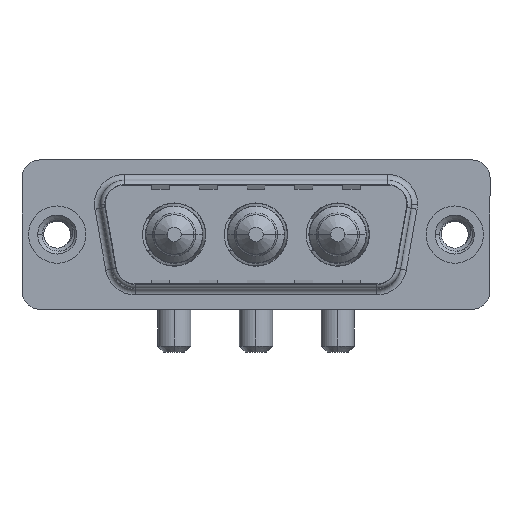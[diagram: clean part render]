
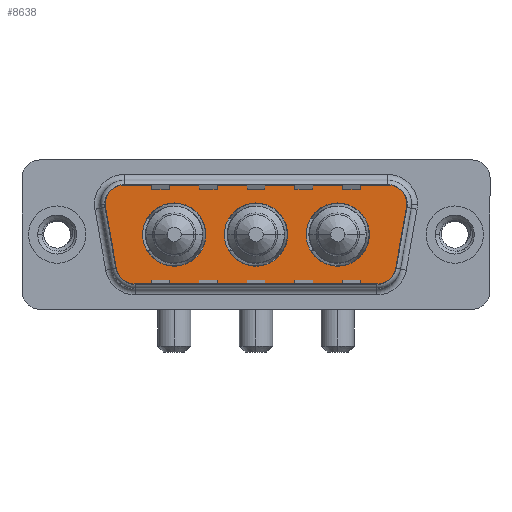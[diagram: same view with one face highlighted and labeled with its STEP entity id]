
A CAD part, top view. The second image highlights one B-rep face of the part: STEP entity #8638.
In plain terms, the highlighted planar face has unit normal (0, 0, 1).
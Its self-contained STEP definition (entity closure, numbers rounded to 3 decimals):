
#4 = CARTESIAN_POINT ( 'NONE',  ( 5.411, 2.9, 0. ) ) ;
#102 = EDGE_CURVE ( 'NONE', #4519, #10215, #9988, .T. ) ;
#134 = CARTESIAN_POINT ( 'NONE',  ( 5.411, 4.9, 0. ) ) ;
#168 = DIRECTION ( 'NONE',  ( 1., 0., 0. ) ) ;
#295 = CIRCLE ( 'NONE', #10770, 2. ) ;
#308 = DIRECTION ( 'NONE',  ( 1., 0., 0. ) ) ;
#319 = LINE ( 'NONE', #379, #3929 ) ;
#379 = CARTESIAN_POINT ( 'NONE',  ( 3.441, 2.553, 0. ) ) ;
#407 = EDGE_LOOP ( 'NONE', ( #12001, #1550 ) ) ;
#461 = EDGE_CURVE ( 'NONE', #5105, #5232, #768, .T. ) ;
#564 = VERTEX_POINT ( 'NONE', #7738 ) ;
#615 = DIRECTION ( 'NONE',  ( 0., 0., 1. ) ) ;
#768 = CIRCLE ( 'NONE', #2025, 2.65 ) ;
#1009 = ORIENTED_EDGE ( 'NONE', *, *, #1290, .T. ) ;
#1150 = CARTESIAN_POINT ( 'NONE',  ( 9.8, 0., 0. ) ) ;
#1290 = EDGE_CURVE ( 'NONE', #6706, #10759, #6469, .T. ) ;
#1369 = EDGE_LOOP ( 'NONE', ( #8035, #1009, #5273, #9855, #12425, #7661, #12326, #8257, #8322 ) ) ;
#1381 = DIRECTION ( 'NONE',  ( 1., 0., 0. ) ) ;
#1436 = DIRECTION ( 'NONE',  ( 1., 0., 0. ) ) ;
#1550 = ORIENTED_EDGE ( 'NONE', *, *, #9164, .F. ) ;
#1664 = CARTESIAN_POINT ( 'NONE',  ( 27.889, 2.9, 0. ) ) ;
#1695 = DIRECTION ( 'NONE',  ( 1., 0., 0. ) ) ;
#1809 = EDGE_CURVE ( 'NONE', #5110, #6706, #10409, .T. ) ;
#2025 = AXIS2_PLACEMENT_3D ( 'NONE', #12736, #9695, #1695 ) ;
#2200 = FACE_BOUND ( 'NONE', #7278, .T. ) ;
#2333 = EDGE_CURVE ( 'NONE', #10215, #7898, #319, .T. ) ;
#2494 = ORIENTED_EDGE ( 'NONE', *, *, #5559, .F. ) ;
#2675 = DIRECTION ( 'NONE',  ( -1., 0., 0. ) ) ;
#2736 = VERTEX_POINT ( 'NONE', #4322 ) ;
#3080 = CARTESIAN_POINT ( 'NONE',  ( 5.411, 4.9, 0. ) ) ;
#3264 = CARTESIAN_POINT ( 'NONE',  ( 26.15, 0., 0. ) ) ;
#3303 = AXIS2_PLACEMENT_3D ( 'NONE', #10310, #6513, #1381 ) ;
#3360 = EDGE_CURVE ( 'NONE', #8669, #5110, #3575, .T. ) ;
#3575 = LINE ( 'NONE', #11386, #5427 ) ;
#3820 = AXIS2_PLACEMENT_3D ( 'NONE', #5224, #9296, #308 ) ;
#3929 = VECTOR ( 'NONE', #7408, 1000. ) ;
#4125 = DIRECTION ( 'NONE',  ( 0., 0., 1. ) ) ;
#4252 = AXIS2_PLACEMENT_3D ( 'NONE', #1150, #4295, #168 ) ;
#4295 = DIRECTION ( 'NONE',  ( 0., 0., 1. ) ) ;
#4322 = CARTESIAN_POINT ( 'NONE',  ( 19.3, 0., 0. ) ) ;
#4519 = VERTEX_POINT ( 'NONE', #3080 ) ;
#4609 = CARTESIAN_POINT ( 'NONE',  ( 6.434, -2.9, 0. ) ) ;
#4753 = AXIS2_PLACEMENT_3D ( 'NONE', #5583, #12183, #9575 ) ;
#4786 = CIRCLE ( 'NONE', #9814, 2. ) ;
#5051 = DIRECTION ( 'NONE',  ( -1., 0., 0. ) ) ;
#5105 = VERTEX_POINT ( 'NONE', #9562 ) ;
#5110 = VERTEX_POINT ( 'NONE', #7670 ) ;
#5224 = CARTESIAN_POINT ( 'NONE',  ( 26.866, -2.9, 0. ) ) ;
#5232 = VERTEX_POINT ( 'NONE', #8582 ) ;
#5273 = ORIENTED_EDGE ( 'NONE', *, *, #9786, .T. ) ;
#5292 = FACE_OUTER_BOUND ( 'NONE', #1369, .T. ) ;
#5427 = VECTOR ( 'NONE', #1436, 1000. ) ;
#5540 = DIRECTION ( 'NONE',  ( 1., 0., 0. ) ) ;
#5559 = EDGE_CURVE ( 'NONE', #5232, #5105, #12180, .T. ) ;
#5583 = CARTESIAN_POINT ( 'NONE',  ( 26.866, -2.9, 0. ) ) ;
#5640 = CIRCLE ( 'NONE', #3303, 2.65 ) ;
#5834 = VECTOR ( 'NONE', #11415, 1000. ) ;
#5925 = CARTESIAN_POINT ( 'NONE',  ( 4.464, -3.247, 0. ) ) ;
#5934 = CIRCLE ( 'NONE', #12594, 2.65 ) ;
#5980 = EDGE_LOOP ( 'NONE', ( #7866, #2494 ) ) ;
#6469 = LINE ( 'NONE', #12451, #5834 ) ;
#6513 = DIRECTION ( 'NONE',  ( 0., 0., 1. ) ) ;
#6523 = DIRECTION ( 'NONE',  ( 1., 0., 0. ) ) ;
#6631 = VERTEX_POINT ( 'NONE', #7946 ) ;
#6706 = VERTEX_POINT ( 'NONE', #8927 ) ;
#6759 = CARTESIAN_POINT ( 'NONE',  ( 3.441, 2.553, 0. ) ) ;
#7204 = FACE_BOUND ( 'NONE', #407, .T. ) ;
#7278 = EDGE_LOOP ( 'NONE', ( #9445, #10167 ) ) ;
#7308 = CIRCLE ( 'NONE', #8562, 2.65 ) ;
#7408 = DIRECTION ( 'NONE',  ( 0.174, -0.985, 0. ) ) ;
#7427 = VERTEX_POINT ( 'NONE', #9729 ) ;
#7497 = DIRECTION ( 'NONE',  ( 0., 0., 1. ) ) ;
#7509 = EDGE_CURVE ( 'NONE', #6631, #7427, #8810, .T. ) ;
#7661 = ORIENTED_EDGE ( 'NONE', *, *, #102, .T. ) ;
#7670 = CARTESIAN_POINT ( 'NONE',  ( 26.866, -4.9, 0. ) ) ;
#7671 = EDGE_CURVE ( 'NONE', #564, #9470, #5934, .T. ) ;
#7738 = CARTESIAN_POINT ( 'NONE',  ( 20.85, 0., 0. ) ) ;
#7797 = EDGE_CURVE ( 'NONE', #7898, #8669, #295, .T. ) ;
#7806 = CARTESIAN_POINT ( 'NONE',  ( 29.859, 2.553, 0. ) ) ;
#7866 = ORIENTED_EDGE ( 'NONE', *, *, #461, .F. ) ;
#7898 = VERTEX_POINT ( 'NONE', #5925 ) ;
#7946 = CARTESIAN_POINT ( 'NONE',  ( 29.889, 2.9, 0. ) ) ;
#8029 = EDGE_CURVE ( 'NONE', #7427, #4519, #11969, .T. ) ;
#8035 = ORIENTED_EDGE ( 'NONE', *, *, #1809, .T. ) ;
#8090 = CARTESIAN_POINT ( 'NONE',  ( 23.5, 0., 0. ) ) ;
#8257 = ORIENTED_EDGE ( 'NONE', *, *, #7797, .T. ) ;
#8322 = ORIENTED_EDGE ( 'NONE', *, *, #3360, .T. ) ;
#8530 = AXIS2_PLACEMENT_3D ( 'NONE', #4, #8993, #11202 ) ;
#8562 = AXIS2_PLACEMENT_3D ( 'NONE', #8090, #4125, #9130 ) ;
#8582 = CARTESIAN_POINT ( 'NONE',  ( 7.15, 0., 0. ) ) ;
#8638 = ADVANCED_FACE ( 'NONE', ( #7204, #2200, #10341, #5292 ), #10208, .T. ) ;
#8669 = VERTEX_POINT ( 'NONE', #12396 ) ;
#8764 = CIRCLE ( 'NONE', #12690, 2.65 ) ;
#8799 = DIRECTION ( 'NONE',  ( 0., 0., 1. ) ) ;
#8810 = CIRCLE ( 'NONE', #9433, 2. ) ;
#8927 = CARTESIAN_POINT ( 'NONE',  ( 28.836, -3.247, 0. ) ) ;
#8993 = DIRECTION ( 'NONE',  ( 0., 0., 1. ) ) ;
#9130 = DIRECTION ( 'NONE',  ( 1., 0., 0. ) ) ;
#9164 = EDGE_CURVE ( 'NONE', #10050, #2736, #8764, .T. ) ;
#9296 = DIRECTION ( 'NONE',  ( 0., 0., 1. ) ) ;
#9433 = AXIS2_PLACEMENT_3D ( 'NONE', #1664, #10719, #11926 ) ;
#9445 = ORIENTED_EDGE ( 'NONE', *, *, #9495, .F. ) ;
#9470 = VERTEX_POINT ( 'NONE', #3264 ) ;
#9495 = EDGE_CURVE ( 'NONE', #9470, #564, #7308, .T. ) ;
#9562 = CARTESIAN_POINT ( 'NONE',  ( 12.45, 0., 0. ) ) ;
#9575 = DIRECTION ( 'NONE',  ( 1., 0., 0. ) ) ;
#9576 = EDGE_CURVE ( 'NONE', #2736, #10050, #5640, .T. ) ;
#9654 = DIRECTION ( 'NONE',  ( -1., 0., 0. ) ) ;
#9695 = DIRECTION ( 'NONE',  ( 0., 0., 1. ) ) ;
#9729 = CARTESIAN_POINT ( 'NONE',  ( 27.889, 4.9, 0. ) ) ;
#9786 = EDGE_CURVE ( 'NONE', #10759, #6631, #4786, .T. ) ;
#9814 = AXIS2_PLACEMENT_3D ( 'NONE', #12686, #8799, #2675 ) ;
#9855 = ORIENTED_EDGE ( 'NONE', *, *, #7509, .T. ) ;
#9988 = CIRCLE ( 'NONE', #8530, 2. ) ;
#10050 = VERTEX_POINT ( 'NONE', #10410 ) ;
#10167 = ORIENTED_EDGE ( 'NONE', *, *, #7671, .F. ) ;
#10208 = PLANE ( 'NONE',  #3820 ) ;
#10215 = VERTEX_POINT ( 'NONE', #6759 ) ;
#10310 = CARTESIAN_POINT ( 'NONE',  ( 16.65, 0., 0. ) ) ;
#10341 = FACE_BOUND ( 'NONE', #5980, .T. ) ;
#10409 = CIRCLE ( 'NONE', #4753, 2. ) ;
#10410 = CARTESIAN_POINT ( 'NONE',  ( 14., 0., 0. ) ) ;
#10445 = CARTESIAN_POINT ( 'NONE',  ( 16.65, 0., 0. ) ) ;
#10719 = DIRECTION ( 'NONE',  ( 0., 0., 1. ) ) ;
#10759 = VERTEX_POINT ( 'NONE', #7806 ) ;
#10770 = AXIS2_PLACEMENT_3D ( 'NONE', #4609, #11530, #9654 ) ;
#11202 = DIRECTION ( 'NONE',  ( 1., 0., 0. ) ) ;
#11279 = CARTESIAN_POINT ( 'NONE',  ( 23.5, 0., 0. ) ) ;
#11386 = CARTESIAN_POINT ( 'NONE',  ( 6.434, -4.9, 0. ) ) ;
#11415 = DIRECTION ( 'NONE',  ( 0.174, 0.985, 0. ) ) ;
#11530 = DIRECTION ( 'NONE',  ( 0., 0., 1. ) ) ;
#11926 = DIRECTION ( 'NONE',  ( -1., 0., 0. ) ) ;
#11969 = LINE ( 'NONE', #134, #12043 ) ;
#12001 = ORIENTED_EDGE ( 'NONE', *, *, #9576, .F. ) ;
#12043 = VECTOR ( 'NONE', #5051, 1000. ) ;
#12180 = CIRCLE ( 'NONE', #4252, 2.65 ) ;
#12183 = DIRECTION ( 'NONE',  ( 0., 0., 1. ) ) ;
#12326 = ORIENTED_EDGE ( 'NONE', *, *, #2333, .T. ) ;
#12396 = CARTESIAN_POINT ( 'NONE',  ( 6.434, -4.9, 0. ) ) ;
#12425 = ORIENTED_EDGE ( 'NONE', *, *, #8029, .T. ) ;
#12451 = CARTESIAN_POINT ( 'NONE',  ( 29.859, 2.553, 0. ) ) ;
#12594 = AXIS2_PLACEMENT_3D ( 'NONE', #11279, #7497, #6523 ) ;
#12686 = CARTESIAN_POINT ( 'NONE',  ( 27.889, 2.9, 0. ) ) ;
#12690 = AXIS2_PLACEMENT_3D ( 'NONE', #10445, #615, #5540 ) ;
#12736 = CARTESIAN_POINT ( 'NONE',  ( 9.8, 0., 0. ) ) ;
